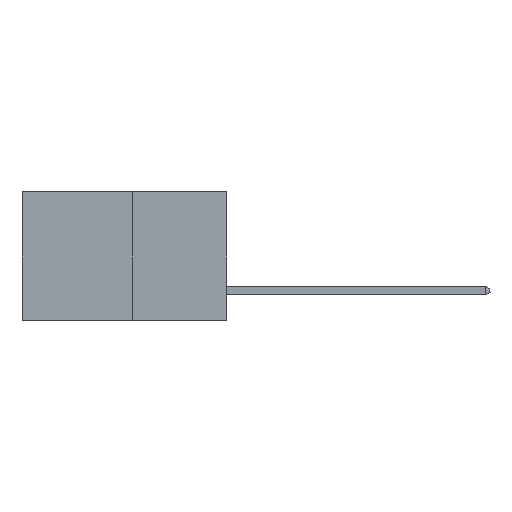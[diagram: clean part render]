
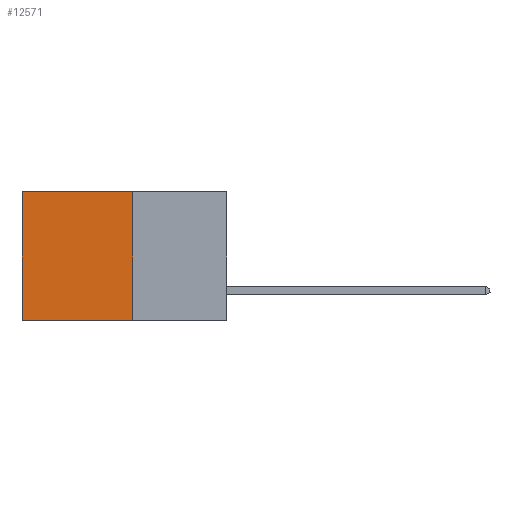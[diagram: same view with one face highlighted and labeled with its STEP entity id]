
A CAD part, left-side view. The second image highlights one B-rep face of the part: STEP entity #12571.
In plain terms, the highlighted planar face has unit normal (-1, 0, 0).
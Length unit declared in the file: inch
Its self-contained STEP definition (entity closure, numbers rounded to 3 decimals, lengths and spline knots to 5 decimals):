
#797 = VECTOR ( 'NONE', #31799, 39.37008 ) ;
#1657 = CARTESIAN_POINT ( 'NONE',  ( 0.277, 0.27, -0.37 ) ) ;
#2234 = CARTESIAN_POINT ( 'NONE',  ( 0.277, 0.27, 0. ) ) ;
#4636 = VERTEX_POINT ( 'NONE', #2234 ) ;
#4985 = CARTESIAN_POINT ( 'NONE',  ( 0.277, 0.27, -0.37 ) ) ;
#5794 = CARTESIAN_POINT ( 'NONE',  ( 0.277, 0.59, -0.37 ) ) ;
#6640 = DIRECTION ( 'NONE',  ( 0., 1., 0. ) ) ;
#8142 = CARTESIAN_POINT ( 'NONE',  ( 0.277, 0.59, -0.37 ) ) ;
#8314 = DIRECTION ( 'NONE',  ( 0., 0., -1. ) ) ;
#11137 = ORIENTED_EDGE ( 'NONE', *, *, #13693, .F. ) ;
#11220 = DIRECTION ( 'NONE',  ( 1., 0., 0. ) ) ;
#12479 = ORIENTED_EDGE ( 'NONE', *, *, #28793, .T. ) ;
#12571 = ADVANCED_FACE ( 'NONE', ( #22941 ), #30043, .F. ) ;
#12832 = LINE ( 'NONE', #13651, #18718 ) ;
#13651 = CARTESIAN_POINT ( 'NONE',  ( 0.277, 0.27, 0. ) ) ;
#13693 = EDGE_CURVE ( 'NONE', #4636, #23051, #15071, .T. ) ;
#14883 = CARTESIAN_POINT ( 'NONE',  ( 0.277, 0.27, -0.37 ) ) ;
#15071 = LINE ( 'NONE', #29343, #797 ) ;
#17049 = VERTEX_POINT ( 'NONE', #8142 ) ;
#17659 = DIRECTION ( 'NONE',  ( 0., 0., -1. ) ) ;
#18718 = VECTOR ( 'NONE', #28597, 39.37008 ) ;
#20838 = VERTEX_POINT ( 'NONE', #21103 ) ;
#20864 = EDGE_CURVE ( 'NONE', #4636, #20838, #12832, .T. ) ;
#21103 = CARTESIAN_POINT ( 'NONE',  ( 0.277, 0.59, 0. ) ) ;
#21964 = EDGE_LOOP ( 'NONE', ( #12479, #26240, #11137, #24227 ) ) ;
#22941 = FACE_OUTER_BOUND ( 'NONE', #21964, .T. ) ;
#23051 = VERTEX_POINT ( 'NONE', #14883 ) ;
#24227 = ORIENTED_EDGE ( 'NONE', *, *, #20864, .T. ) ;
#25092 = VECTOR ( 'NONE', #8314, 39.37008 ) ;
#25357 = AXIS2_PLACEMENT_3D ( 'NONE', #4985, #11220, #17659 ) ;
#25874 = LINE ( 'NONE', #5794, #25092 ) ;
#26240 = ORIENTED_EDGE ( 'NONE', *, *, #30369, .F. ) ;
#28084 = LINE ( 'NONE', #1657, #28853 ) ;
#28597 = DIRECTION ( 'NONE',  ( 0., 1., 0. ) ) ;
#28793 = EDGE_CURVE ( 'NONE', #20838, #17049, #25874, .T. ) ;
#28853 = VECTOR ( 'NONE', #6640, 39.37008 ) ;
#29343 = CARTESIAN_POINT ( 'NONE',  ( 0.277, 0.27, -0.37 ) ) ;
#30043 = PLANE ( 'NONE',  #25357 ) ;
#30369 = EDGE_CURVE ( 'NONE', #23051, #17049, #28084, .T. ) ;
#31799 = DIRECTION ( 'NONE',  ( 0., 0., -1. ) ) ;
